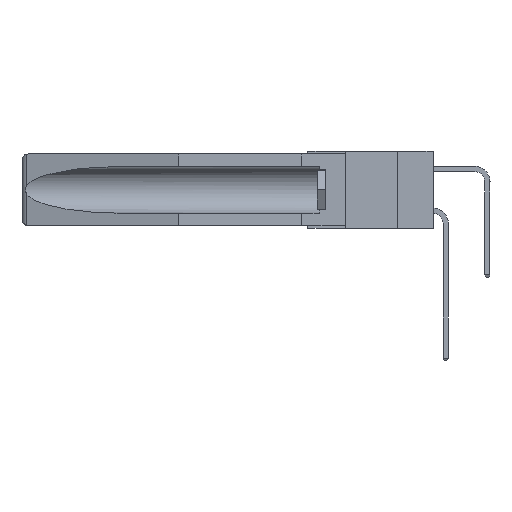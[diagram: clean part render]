
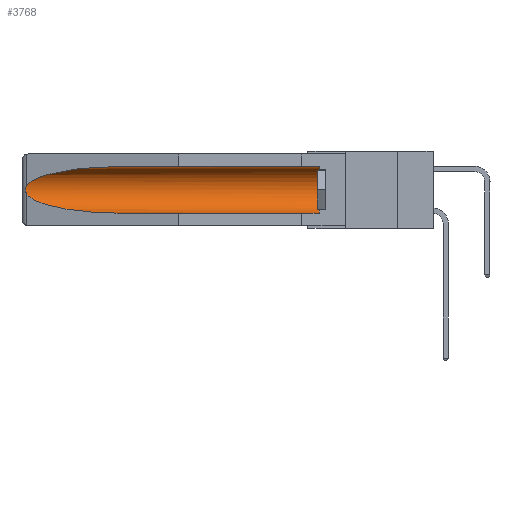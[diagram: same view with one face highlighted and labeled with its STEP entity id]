
A CAD part, left-side view. The second image highlights one B-rep face of the part: STEP entity #3768.
In plain terms, the highlighted cylindrical face has radius 2.857 mm (diameter 5.715 mm), a partial arc.
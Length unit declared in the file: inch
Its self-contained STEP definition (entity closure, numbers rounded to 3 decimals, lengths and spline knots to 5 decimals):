
#652 = AXIS2_PLACEMENT_3D ( 'NONE', #30650, #20685, #22979 ) ;
#2076 = CARTESIAN_POINT ( 'NONE',  ( 0.26597, 1.52961, -0.15275 ) ) ;
#2229 = DIRECTION ( 'NONE',  ( 0., 1., 0. ) ) ;
#2264 = CARTESIAN_POINT ( 'NONE',  ( 0.26537, 1.52718, -0.19328 ) ) ;
#2471 = CARTESIAN_POINT ( 'NONE',  ( 0.21114, 1.30732, -0.059 ) ) ;
#2582 = EDGE_CURVE ( 'NONE', #12855, #13861, #14323, .T. ) ;
#2927 = CARTESIAN_POINT ( 'NONE',  ( 0.25451, 1.48313, -0.24835 ) ) ;
#2951 = ORIENTED_EDGE ( 'NONE', *, *, #17331, .T. ) ;
#3768 = ADVANCED_FACE ( 'NONE', ( #19197 ), #11698, .F. ) ;
#4532 = CARTESIAN_POINT ( 'NONE',  ( 0.26537, 1.52718, -0.14972 ) ) ;
#4855 = CARTESIAN_POINT ( 'NONE',  ( 0.155, 1.07973, -0.059 ) ) ;
#5162 =( BOUNDED_CURVE ( )  B_SPLINE_CURVE ( 3, ( #7716, #2927, #25254, #20443 ),
 .UNSPECIFIED., .F., .T. ) 
 B_SPLINE_CURVE_WITH_KNOTS ( ( 4, 4 ),
 ( 0.1948, 1.5708 ),
 .UNSPECIFIED. ) 
 CURVE ( )  GEOMETRIC_REPRESENTATION_ITEM ( )  RATIONAL_B_SPLINE_CURVE ( ( 1., 0.848, 0.848, 1. ) ) 
 REPRESENTATION_ITEM ( '' )  );
#6054 = EDGE_CURVE ( 'NONE', #28193, #24654, #20149, .T. ) ;
#7716 = CARTESIAN_POINT ( 'NONE',  ( 0.26537, 1.52718, -0.19328 ) ) ;
#8357 = CARTESIAN_POINT ( 'NONE',  ( 0.155, 0.126, -0.284 ) ) ;
#8591 = ORIENTED_EDGE ( 'NONE', *, *, #29609, .F. ) ;
#9215 = CARTESIAN_POINT ( 'NONE',  ( 0.2673, 1.5327, -0.16383 ) ) ;
#10099 = CARTESIAN_POINT ( 'NONE',  ( 0.2675, 1.53308, -0.17534 ) ) ;
#11055 = ORIENTED_EDGE ( 'NONE', *, *, #2582, .T. ) ;
#11363 = CARTESIAN_POINT ( 'NONE',  ( 0.155, -0.30754, -0.059 ) ) ;
#11698 = CYLINDRICAL_SURFACE ( 'NONE', #13407, 0.1125 ) ;
#12177 = CARTESIAN_POINT ( 'NONE',  ( 0.26655, 1.53094, -0.18657 ) ) ;
#12855 = VERTEX_POINT ( 'NONE', #16720 ) ;
#13407 = AXIS2_PLACEMENT_3D ( 'NONE', #15328, #17830, #20096 ) ;
#13861 = VERTEX_POINT ( 'NONE', #15578 ) ;
#14323 =( BOUNDED_CURVE ( )  B_SPLINE_CURVE ( 3, ( #4855, #2471, #27226, #4532 ),
 .UNSPECIFIED., .F., .T. ) 
 B_SPLINE_CURVE_WITH_KNOTS ( ( 4, 4 ),
 ( 4.71239, 6.08839 ),
 .UNSPECIFIED. ) 
 CURVE ( )  GEOMETRIC_REPRESENTATION_ITEM ( )  RATIONAL_B_SPLINE_CURVE ( ( 1., 0.848, 0.848, 1. ) ) 
 REPRESENTATION_ITEM ( '' )  );
#14566 = EDGE_CURVE ( 'NONE', #21098, #27131, #5162, .T. ) ;
#15328 = CARTESIAN_POINT ( 'NONE',  ( 0.155, -0.30754, -0.1715 ) ) ;
#15578 = CARTESIAN_POINT ( 'NONE',  ( 0.26537, 1.52718, -0.14972 ) ) ;
#16720 = CARTESIAN_POINT ( 'NONE',  ( 0.155, 1.07973, -0.059 ) ) ;
#16797 = CARTESIAN_POINT ( 'NONE',  ( 0.155, -0.30754, -0.284 ) ) ;
#17331 = EDGE_CURVE ( 'NONE', #13861, #21098, #20630, .T. ) ;
#17664 = LINE ( 'NONE', #11363, #26673 ) ;
#17830 = DIRECTION ( 'NONE',  ( 0., 1., 0. ) ) ;
#19197 = FACE_OUTER_BOUND ( 'NONE', #24894, .T. ) ;
#20096 = DIRECTION ( 'NONE',  ( 0., 0., 1. ) ) ;
#20149 = CIRCLE ( 'NONE', #652, 0.1125 ) ;
#20409 = ORIENTED_EDGE ( 'NONE', *, *, #14566, .T. ) ;
#20443 = CARTESIAN_POINT ( 'NONE',  ( 0.155, 1.07973, -0.284 ) ) ;
#20630 = B_SPLINE_CURVE_WITH_KNOTS ( 'NONE', 3,
 ( #32081, #2076, #22391, #9215, #22453, #10099, #31042, #12177, #27391, #27606 ),
 .UNSPECIFIED., .F., .F.,
 ( 4, 2, 2, 2, 4 ),
 ( 0., 0.00029, 0.00058, 0.00087, 0.00117 ),
 .UNSPECIFIED. ) ;
#20685 = DIRECTION ( 'NONE',  ( 0., -1., 0. ) ) ;
#21098 = VERTEX_POINT ( 'NONE', #2264 ) ;
#22391 = CARTESIAN_POINT ( 'NONE',  ( 0.26654, 1.53092, -0.15636 ) ) ;
#22453 = CARTESIAN_POINT ( 'NONE',  ( 0.2675, 1.53308, -0.16763 ) ) ;
#22949 = ORIENTED_EDGE ( 'NONE', *, *, #6054, .T. ) ;
#22979 = DIRECTION ( 'NONE',  ( 0., 0., 1. ) ) ;
#23174 = CARTESIAN_POINT ( 'NONE',  ( 0.155, 1.07973, -0.284 ) ) ;
#23466 = VECTOR ( 'NONE', #2229, 39.37008 ) ;
#24510 = CARTESIAN_POINT ( 'NONE',  ( 0.155, 0.126, -0.059 ) ) ;
#24654 = VERTEX_POINT ( 'NONE', #24510 ) ;
#24894 = EDGE_LOOP ( 'NONE', ( #11055, #2951, #20409, #8591, #22949, #28496 ) ) ;
#25254 = CARTESIAN_POINT ( 'NONE',  ( 0.21114, 1.30732, -0.284 ) ) ;
#26496 = DIRECTION ( 'NONE',  ( 0., 1., 0. ) ) ;
#26673 = VECTOR ( 'NONE', #26496, 39.37008 ) ;
#27131 = VERTEX_POINT ( 'NONE', #23174 ) ;
#27226 = CARTESIAN_POINT ( 'NONE',  ( 0.25451, 1.48313, -0.09465 ) ) ;
#27391 = CARTESIAN_POINT ( 'NONE',  ( 0.26597, 1.5296, -0.19026 ) ) ;
#27606 = CARTESIAN_POINT ( 'NONE',  ( 0.26537, 1.52718, -0.19328 ) ) ;
#28193 = VERTEX_POINT ( 'NONE', #8357 ) ;
#28496 = ORIENTED_EDGE ( 'NONE', *, *, #29179, .T. ) ;
#29179 = EDGE_CURVE ( 'NONE', #24654, #12855, #17664, .T. ) ;
#29609 = EDGE_CURVE ( 'NONE', #28193, #27131, #30145, .T. ) ;
#30145 = LINE ( 'NONE', #16797, #23466 ) ;
#30650 = CARTESIAN_POINT ( 'NONE',  ( 0.155, 0.126, -0.1715 ) ) ;
#31042 = CARTESIAN_POINT ( 'NONE',  ( 0.2673, 1.53269, -0.17917 ) ) ;
#32081 = CARTESIAN_POINT ( 'NONE',  ( 0.26537, 1.52718, -0.14972 ) ) ;
